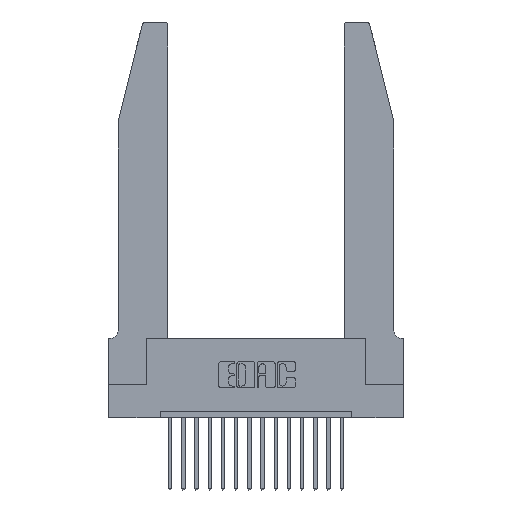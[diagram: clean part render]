
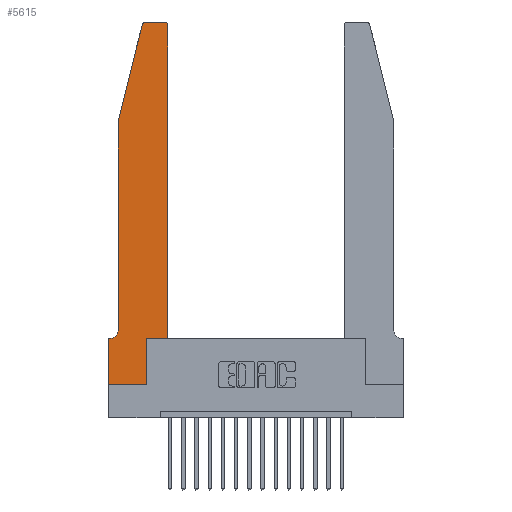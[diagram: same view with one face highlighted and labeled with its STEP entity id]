
A CAD part, top view. The second image highlights one B-rep face of the part: STEP entity #5615.
In plain terms, the highlighted planar face has unit normal (0, 0, 1).
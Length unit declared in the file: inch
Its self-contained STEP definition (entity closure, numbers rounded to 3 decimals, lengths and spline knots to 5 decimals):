
#188 = LINE ( 'NONE', #6587, #5071 ) ;
#568 = DIRECTION ( 'NONE',  ( 1., 0., 0. ) ) ;
#683 = CIRCLE ( 'NONE', #10922, 0.03 ) ;
#732 = CARTESIAN_POINT ( 'NONE',  ( 0.4205, 2.72, 0.37 ) ) ;
#1346 = EDGE_CURVE ( 'NONE', #10544, #5289, #12059, .T. ) ;
#1520 = CARTESIAN_POINT ( 'NONE',  ( 0.284, 2.75, 0.37 ) ) ;
#1758 = VERTEX_POINT ( 'NONE', #1520 ) ;
#1910 = CARTESIAN_POINT ( 'NONE',  ( 0.0055, 0.42, 0.37 ) ) ;
#3342 = CARTESIAN_POINT ( 'NONE',  ( 0.2865, 0., 0.37 ) ) ;
#3413 = ORIENTED_EDGE ( 'NONE', *, *, #9256, .T. ) ;
#3436 = FACE_OUTER_BOUND ( 'NONE', #18198, .T. ) ;
#3785 = DIRECTION ( 'NONE',  ( -0.239, -0.971, 0. ) ) ;
#4022 = CARTESIAN_POINT ( 'NONE',  ( 0.4505, 2.72, 0.37 ) ) ;
#4718 = CARTESIAN_POINT ( 'NONE',  ( 0.25487, 2.72718, 0.37 ) ) ;
#4736 = CARTESIAN_POINT ( 'NONE',  ( 0.2865, 0.35, 0.37 ) ) ;
#4855 = DIRECTION ( 'NONE',  ( 1., 0., 0. ) ) ;
#4872 = EDGE_CURVE ( 'NONE', #10798, #10544, #15694, .T. ) ;
#4932 = VECTOR ( 'NONE', #9386, 39.37008 ) ;
#4995 = EDGE_CURVE ( 'NONE', #5106, #6973, #683, .T. ) ;
#5030 = CARTESIAN_POINT ( 'NONE',  ( 0., 0., 0.37 ) ) ;
#5034 = DIRECTION ( 'NONE',  ( 0., 0., 1. ) ) ;
#5071 = VECTOR ( 'NONE', #8071, 39.37008 ) ;
#5106 = VERTEX_POINT ( 'NONE', #4022 ) ;
#5289 = VERTEX_POINT ( 'NONE', #17367 ) ;
#5310 = LINE ( 'NONE', #6730, #11801 ) ;
#5490 = ORIENTED_EDGE ( 'NONE', *, *, #15712, .T. ) ;
#5615 = ADVANCED_FACE ( 'NONE', ( #3436 ), #18196, .T. ) ;
#5831 = ORIENTED_EDGE ( 'NONE', *, *, #1346, .T. ) ;
#6173 = ORIENTED_EDGE ( 'NONE', *, *, #14359, .T. ) ;
#6411 = CIRCLE ( 'NONE', #8210, 0.03 ) ;
#6587 = CARTESIAN_POINT ( 'NONE',  ( 0., 0., 0.37 ) ) ;
#6603 = LINE ( 'NONE', #14785, #14886 ) ;
#6730 = CARTESIAN_POINT ( 'NONE',  ( 0.4505, 0.35, 0.37 ) ) ;
#6973 = VERTEX_POINT ( 'NONE', #14495 ) ;
#7005 = ORIENTED_EDGE ( 'NONE', *, *, #17703, .T. ) ;
#7067 = EDGE_CURVE ( 'NONE', #6973, #1758, #11971, .T. ) ;
#7166 = CARTESIAN_POINT ( 'NONE',  ( 0.0055, 0.35, 0.37 ) ) ;
#7191 = CARTESIAN_POINT ( 'NONE',  ( 0.2605, 2.75, 0.37 ) ) ;
#7717 = DIRECTION ( 'NONE',  ( 0., 1., 0. ) ) ;
#7821 = DIRECTION ( 'NONE',  ( 0., 0., -1. ) ) ;
#7888 = DIRECTION ( 'NONE',  ( 0., 0., 1. ) ) ;
#7904 = ORIENTED_EDGE ( 'NONE', *, *, #18525, .T. ) ;
#8055 = CARTESIAN_POINT ( 'NONE',  ( 0.0755, 2., 0.37 ) ) ;
#8071 = DIRECTION ( 'NONE',  ( 1., 0., 0. ) ) ;
#8115 = VECTOR ( 'NONE', #3785, 39.37008 ) ;
#8129 = DIRECTION ( 'NONE',  ( 1., 0., 0. ) ) ;
#8210 = AXIS2_PLACEMENT_3D ( 'NONE', #16652, #7888, #568 ) ;
#8856 = ORIENTED_EDGE ( 'NONE', *, *, #4995, .T. ) ;
#8971 = CIRCLE ( 'NONE', #18306, 0.07 ) ;
#9217 = CARTESIAN_POINT ( 'NONE',  ( 0., 0.35, 0.37 ) ) ;
#9256 = EDGE_CURVE ( 'NONE', #16461, #17183, #9807, .T. ) ;
#9386 = DIRECTION ( 'NONE',  ( 0., -1., 0. ) ) ;
#9426 = CARTESIAN_POINT ( 'NONE',  ( 0.4505, 0.35, 0.37 ) ) ;
#9807 = LINE ( 'NONE', #5030, #4932 ) ;
#10291 = CARTESIAN_POINT ( 'NONE',  ( 0., 0., 0.37 ) ) ;
#10544 = VERTEX_POINT ( 'NONE', #18748 ) ;
#10773 = DIRECTION ( 'NONE',  ( -1., 0., 0. ) ) ;
#10798 = VERTEX_POINT ( 'NONE', #3342 ) ;
#10837 = CARTESIAN_POINT ( 'NONE',  ( 0., 0.35, 0.37 ) ) ;
#10879 = LINE ( 'NONE', #8055, #8115 ) ;
#10922 = AXIS2_PLACEMENT_3D ( 'NONE', #732, #5034, #8129 ) ;
#11068 = DIRECTION ( 'NONE',  ( 0., 1., 0. ) ) ;
#11078 = VECTOR ( 'NONE', #18957, 39.37008 ) ;
#11801 = VECTOR ( 'NONE', #11068, 39.37008 ) ;
#11806 = VECTOR ( 'NONE', #7717, 39.37008 ) ;
#11971 = LINE ( 'NONE', #7191, #13792 ) ;
#12059 = LINE ( 'NONE', #9426, #18476 ) ;
#12169 = DIRECTION ( 'NONE',  ( 0., 0., 1. ) ) ;
#12553 = EDGE_CURVE ( 'NONE', #16315, #15340, #10879, .T. ) ;
#13479 = ORIENTED_EDGE ( 'NONE', *, *, #13599, .T. ) ;
#13599 = EDGE_CURVE ( 'NONE', #14654, #16003, #8971, .T. ) ;
#13792 = VECTOR ( 'NONE', #18949, 39.37008 ) ;
#13835 = LINE ( 'NONE', #17692, #11078 ) ;
#14089 = ORIENTED_EDGE ( 'NONE', *, *, #7067, .T. ) ;
#14359 = EDGE_CURVE ( 'NONE', #17183, #10798, #188, .T. ) ;
#14495 = CARTESIAN_POINT ( 'NONE',  ( 0.4205, 2.75, 0.37 ) ) ;
#14621 = AXIS2_PLACEMENT_3D ( 'NONE', #9217, #12169, #4855 ) ;
#14654 = VERTEX_POINT ( 'NONE', #17681 ) ;
#14674 = ORIENTED_EDGE ( 'NONE', *, *, #4872, .T. ) ;
#14785 = CARTESIAN_POINT ( 'NONE',  ( 0.0755, 2., 0.37 ) ) ;
#14886 = VECTOR ( 'NONE', #17659, 39.37008 ) ;
#15007 = ORIENTED_EDGE ( 'NONE', *, *, #16763, .T. ) ;
#15340 = VERTEX_POINT ( 'NONE', #15956 ) ;
#15694 = LINE ( 'NONE', #4736, #11806 ) ;
#15712 = EDGE_CURVE ( 'NONE', #1758, #16315, #6411, .T. ) ;
#15956 = CARTESIAN_POINT ( 'NONE',  ( 0.0755, 2., 0.37 ) ) ;
#16003 = VERTEX_POINT ( 'NONE', #7166 ) ;
#16315 = VERTEX_POINT ( 'NONE', #4718 ) ;
#16461 = VERTEX_POINT ( 'NONE', #10837 ) ;
#16482 = ORIENTED_EDGE ( 'NONE', *, *, #12553, .T. ) ;
#16652 = CARTESIAN_POINT ( 'NONE',  ( 0.284, 2.72, 0.37 ) ) ;
#16763 = EDGE_CURVE ( 'NONE', #15340, #14654, #6603, .T. ) ;
#17183 = VERTEX_POINT ( 'NONE', #10291 ) ;
#17367 = CARTESIAN_POINT ( 'NONE',  ( 0.4505, 0.35, 0.37 ) ) ;
#17659 = DIRECTION ( 'NONE',  ( 0., -1., 0. ) ) ;
#17681 = CARTESIAN_POINT ( 'NONE',  ( 0.0755, 0.42, 0.37 ) ) ;
#17692 = CARTESIAN_POINT ( 'NONE',  ( 0.0755, 0.35, 0.37 ) ) ;
#17703 = EDGE_CURVE ( 'NONE', #5289, #5106, #5310, .T. ) ;
#18196 = PLANE ( 'NONE',  #14621 ) ;
#18198 = EDGE_LOOP ( 'NONE', ( #14089, #5490, #16482, #15007, #13479, #7904, #3413, #6173, #14674, #5831, #7005, #8856 ) ) ;
#18306 = AXIS2_PLACEMENT_3D ( 'NONE', #1910, #7821, #10773 ) ;
#18341 = DIRECTION ( 'NONE',  ( 1., 0., 0. ) ) ;
#18476 = VECTOR ( 'NONE', #18341, 39.37008 ) ;
#18525 = EDGE_CURVE ( 'NONE', #16003, #16461, #13835, .T. ) ;
#18748 = CARTESIAN_POINT ( 'NONE',  ( 0.2865, 0.35, 0.37 ) ) ;
#18949 = DIRECTION ( 'NONE',  ( -1., 0., 0. ) ) ;
#18957 = DIRECTION ( 'NONE',  ( -1., 0., 0. ) ) ;
